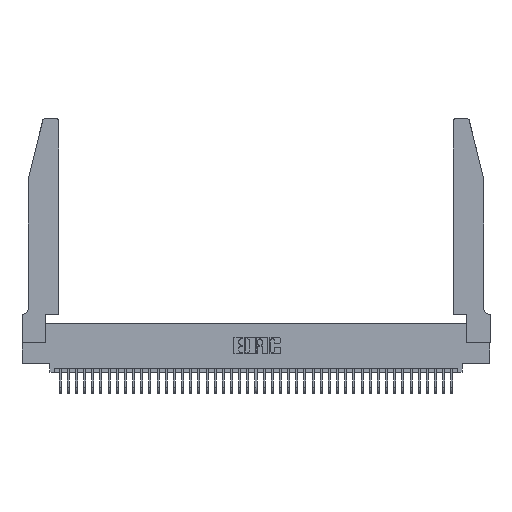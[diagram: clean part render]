
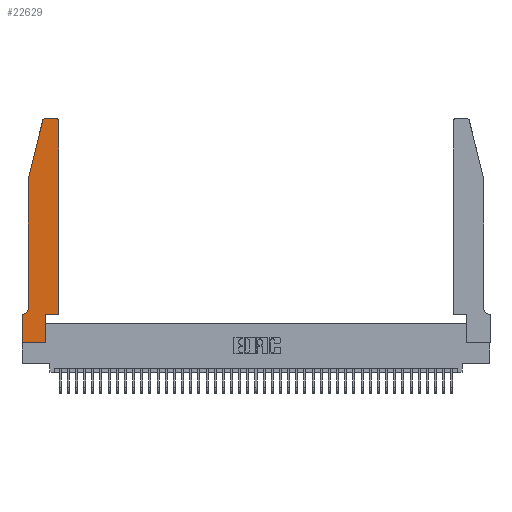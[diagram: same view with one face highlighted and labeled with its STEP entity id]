
A CAD part, top view. The second image highlights one B-rep face of the part: STEP entity #22629.
In plain terms, the highlighted planar face has unit normal (0, 0, 1).
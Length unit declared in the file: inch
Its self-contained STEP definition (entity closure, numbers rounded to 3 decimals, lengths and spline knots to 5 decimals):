
#441 = EDGE_LOOP ( 'NONE', ( #32714, #4043, #14583, #6883, #27617, #30067, #14280, #8827, #23767, #6738, #22883, #2865 ) ) ;
#769 = AXIS2_PLACEMENT_3D ( 'NONE', #42856, #5847, #22546 ) ;
#1963 = CIRCLE ( 'NONE', #5909, 0.03 ) ;
#2351 = EDGE_CURVE ( 'NONE', #9090, #39182, #42327, .T. ) ;
#2553 = EDGE_CURVE ( 'NONE', #10510, #35224, #19440, .T. ) ;
#2655 = CARTESIAN_POINT ( 'NONE',  ( 0.0055, 0.35, 0.37 ) ) ;
#2726 = FACE_OUTER_BOUND ( 'NONE', #441, .T. ) ;
#2865 = ORIENTED_EDGE ( 'NONE', *, *, #34799, .T. ) ;
#3065 = CIRCLE ( 'NONE', #10716, 0.03 ) ;
#3258 = CARTESIAN_POINT ( 'NONE',  ( 0., 0., 0.37 ) ) ;
#4043 = ORIENTED_EDGE ( 'NONE', *, *, #10944, .T. ) ;
#4462 = LINE ( 'NONE', #41244, #41198 ) ;
#5482 = DIRECTION ( 'NONE',  ( -0.239, -0.971, 0. ) ) ;
#5847 = DIRECTION ( 'NONE',  ( 0., 0., 1. ) ) ;
#5909 = AXIS2_PLACEMENT_3D ( 'NONE', #35533, #15136, #38927 ) ;
#6738 = ORIENTED_EDGE ( 'NONE', *, *, #37125, .T. ) ;
#6883 = ORIENTED_EDGE ( 'NONE', *, *, #36104, .T. ) ;
#7356 = CARTESIAN_POINT ( 'NONE',  ( 0., 0.35, 0.37 ) ) ;
#7800 = DIRECTION ( 'NONE',  ( -1., 0., 0. ) ) ;
#8032 = DIRECTION ( 'NONE',  ( -1., 0., 0. ) ) ;
#8514 = CARTESIAN_POINT ( 'NONE',  ( 0.0755, 0.42, 0.37 ) ) ;
#8827 = ORIENTED_EDGE ( 'NONE', *, *, #25747, .T. ) ;
#9042 = DIRECTION ( 'NONE',  ( 1., 0., 0. ) ) ;
#9090 = VERTEX_POINT ( 'NONE', #7356 ) ;
#9540 = VERTEX_POINT ( 'NONE', #29915 ) ;
#10510 = VERTEX_POINT ( 'NONE', #18808 ) ;
#10716 = AXIS2_PLACEMENT_3D ( 'NONE', #11728, #22152, #42482 ) ;
#10944 = EDGE_CURVE ( 'NONE', #42185, #33211, #1963, .T. ) ;
#11728 = CARTESIAN_POINT ( 'NONE',  ( 0.4205, 2.72, 0.37 ) ) ;
#12852 = CARTESIAN_POINT ( 'NONE',  ( 0.2865, 0., 0.37 ) ) ;
#14280 = ORIENTED_EDGE ( 'NONE', *, *, #2351, .T. ) ;
#14583 = ORIENTED_EDGE ( 'NONE', *, *, #29932, .T. ) ;
#14623 = CARTESIAN_POINT ( 'NONE',  ( 0.0055, 0.42, 0.37 ) ) ;
#15136 = DIRECTION ( 'NONE',  ( 0., 0., 1. ) ) ;
#15251 = VERTEX_POINT ( 'NONE', #35574 ) ;
#16436 = VECTOR ( 'NONE', #36011, 39.37008 ) ;
#16474 = CARTESIAN_POINT ( 'NONE',  ( 0.0755, 2., 0.37 ) ) ;
#17641 = LINE ( 'NONE', #39790, #35763 ) ;
#17772 = DIRECTION ( 'NONE',  ( 0., 0., -1. ) ) ;
#17995 = EDGE_CURVE ( 'NONE', #24712, #42185, #39215, .T. ) ;
#18425 = LINE ( 'NONE', #36850, #29112 ) ;
#18808 = CARTESIAN_POINT ( 'NONE',  ( 0.4505, 0.35, 0.37 ) ) ;
#19179 = CARTESIAN_POINT ( 'NONE',  ( 0.4505, 0.35, 0.37 ) ) ;
#19196 = CARTESIAN_POINT ( 'NONE',  ( 0.2865, 0.35, 0.37 ) ) ;
#19440 = LINE ( 'NONE', #19179, #20545 ) ;
#20252 = DIRECTION ( 'NONE',  ( 1., 0., 0. ) ) ;
#20545 = VECTOR ( 'NONE', #32626, 39.37008 ) ;
#21028 = LINE ( 'NONE', #22489, #29547 ) ;
#21572 = VECTOR ( 'NONE', #22933, 39.37008 ) ;
#22152 = DIRECTION ( 'NONE',  ( 0., 0., 1. ) ) ;
#22254 = EDGE_CURVE ( 'NONE', #38191, #29120, #24068, .T. ) ;
#22373 = CARTESIAN_POINT ( 'NONE',  ( 0.2605, 2.75, 0.37 ) ) ;
#22489 = CARTESIAN_POINT ( 'NONE',  ( 0.4505, 0.35, 0.37 ) ) ;
#22546 = DIRECTION ( 'NONE',  ( 1., 0., 0. ) ) ;
#22629 = ADVANCED_FACE ( 'NONE', ( #2726 ), #35748, .T. ) ;
#22883 = ORIENTED_EDGE ( 'NONE', *, *, #2553, .T. ) ;
#22933 = DIRECTION ( 'NONE',  ( 0., -1., 0. ) ) ;
#23540 = CARTESIAN_POINT ( 'NONE',  ( 0., 0., 0.37 ) ) ;
#23767 = ORIENTED_EDGE ( 'NONE', *, *, #40238, .T. ) ;
#24068 = CIRCLE ( 'NONE', #34149, 0.07 ) ;
#24712 = VERTEX_POINT ( 'NONE', #29851 ) ;
#25747 = EDGE_CURVE ( 'NONE', #39182, #41656, #18425, .T. ) ;
#27617 = ORIENTED_EDGE ( 'NONE', *, *, #22254, .T. ) ;
#29112 = VECTOR ( 'NONE', #9042, 39.37008 ) ;
#29120 = VERTEX_POINT ( 'NONE', #2655 ) ;
#29547 = VECTOR ( 'NONE', #20252, 39.37008 ) ;
#29851 = CARTESIAN_POINT ( 'NONE',  ( 0.4205, 2.75, 0.37 ) ) ;
#29915 = CARTESIAN_POINT ( 'NONE',  ( 0.2865, 0.35, 0.37 ) ) ;
#29932 = EDGE_CURVE ( 'NONE', #33211, #15251, #17641, .T. ) ;
#30067 = ORIENTED_EDGE ( 'NONE', *, *, #36264, .T. ) ;
#30192 = CARTESIAN_POINT ( 'NONE',  ( 0.25487, 2.72718, 0.37 ) ) ;
#30258 = VECTOR ( 'NONE', #8032, 39.37008 ) ;
#31764 = VECTOR ( 'NONE', #43555, 39.37008 ) ;
#32626 = DIRECTION ( 'NONE',  ( 0., 1., 0. ) ) ;
#32714 = ORIENTED_EDGE ( 'NONE', *, *, #17995, .T. ) ;
#33211 = VERTEX_POINT ( 'NONE', #30192 ) ;
#34149 = AXIS2_PLACEMENT_3D ( 'NONE', #14623, #17772, #41389 ) ;
#34554 = LINE ( 'NONE', #19196, #16436 ) ;
#34799 = EDGE_CURVE ( 'NONE', #35224, #24712, #3065, .T. ) ;
#34971 = CARTESIAN_POINT ( 'NONE',  ( 0.4505, 2.72, 0.37 ) ) ;
#35224 = VERTEX_POINT ( 'NONE', #34971 ) ;
#35533 = CARTESIAN_POINT ( 'NONE',  ( 0.284, 2.72, 0.37 ) ) ;
#35574 = CARTESIAN_POINT ( 'NONE',  ( 0.0755, 2., 0.37 ) ) ;
#35748 = PLANE ( 'NONE',  #769 ) ;
#35763 = VECTOR ( 'NONE', #5482, 39.37008 ) ;
#36011 = DIRECTION ( 'NONE',  ( 0., 1., 0. ) ) ;
#36104 = EDGE_CURVE ( 'NONE', #15251, #38191, #37495, .T. ) ;
#36264 = EDGE_CURVE ( 'NONE', #29120, #9090, #4462, .T. ) ;
#36850 = CARTESIAN_POINT ( 'NONE',  ( 0., 0., 0.37 ) ) ;
#37125 = EDGE_CURVE ( 'NONE', #9540, #10510, #21028, .T. ) ;
#37495 = LINE ( 'NONE', #16474, #21572 ) ;
#38191 = VERTEX_POINT ( 'NONE', #8514 ) ;
#38927 = DIRECTION ( 'NONE',  ( 1., 0., 0. ) ) ;
#39182 = VERTEX_POINT ( 'NONE', #23540 ) ;
#39215 = LINE ( 'NONE', #22373, #30258 ) ;
#39790 = CARTESIAN_POINT ( 'NONE',  ( 0.0755, 2., 0.37 ) ) ;
#40238 = EDGE_CURVE ( 'NONE', #41656, #9540, #34554, .T. ) ;
#41198 = VECTOR ( 'NONE', #7800, 39.37008 ) ;
#41244 = CARTESIAN_POINT ( 'NONE',  ( 0.0755, 0.35, 0.37 ) ) ;
#41389 = DIRECTION ( 'NONE',  ( -1., 0., 0. ) ) ;
#41656 = VERTEX_POINT ( 'NONE', #12852 ) ;
#42185 = VERTEX_POINT ( 'NONE', #42825 ) ;
#42327 = LINE ( 'NONE', #3258, #31764 ) ;
#42482 = DIRECTION ( 'NONE',  ( 1., 0., 0. ) ) ;
#42825 = CARTESIAN_POINT ( 'NONE',  ( 0.284, 2.75, 0.37 ) ) ;
#42856 = CARTESIAN_POINT ( 'NONE',  ( 0., 0.35, 0.37 ) ) ;
#43555 = DIRECTION ( 'NONE',  ( 0., -1., 0. ) ) ;
